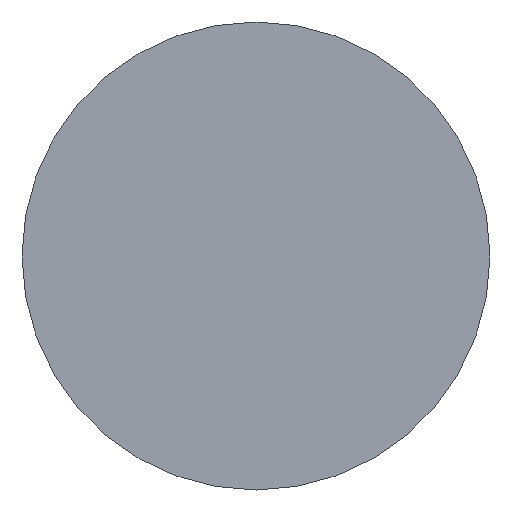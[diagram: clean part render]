
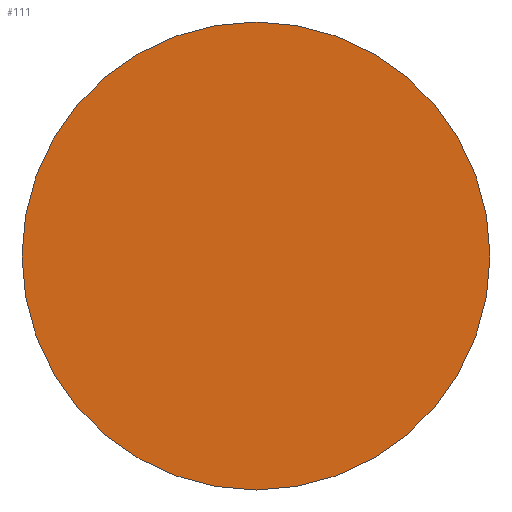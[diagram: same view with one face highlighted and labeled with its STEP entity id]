
A CAD part, left-side view. The second image highlights one B-rep face of the part: STEP entity #111.
In plain terms, the highlighted planar face has unit normal (-1, 0, 0).
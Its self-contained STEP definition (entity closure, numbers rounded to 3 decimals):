
#5 = DIRECTION ( 'NONE',  ( 1., 0., 0. ) ) ;
#15 = DIRECTION ( 'NONE',  ( 1., 0., 0. ) ) ;
#19 = CARTESIAN_POINT ( 'NONE',  ( -418.672, 34.658, 21.5 ) ) ;
#20 = CIRCLE ( 'NONE', #144, 3. ) ;
#22 = DIRECTION ( 'NONE',  ( 0., 0., 1. ) ) ;
#29 = VERTEX_POINT ( 'NONE', #68 ) ;
#35 = DIRECTION ( 'NONE',  ( -1., 0., 0. ) ) ;
#36 = AXIS2_PLACEMENT_3D ( 'NONE', #19, #5, #22 ) ;
#44 = EDGE_LOOP ( 'NONE', ( #69, #57 ) ) ;
#57 = ORIENTED_EDGE ( 'NONE', *, *, #66, .F. ) ;
#60 = PLANE ( 'NONE',  #78 ) ;
#66 = EDGE_CURVE ( 'NONE', #29, #102, #20, .T. ) ;
#68 = CARTESIAN_POINT ( 'NONE',  ( -418.672, 34.658, 18.5 ) ) ;
#69 = ORIENTED_EDGE ( 'NONE', *, *, #104, .F. ) ;
#78 = AXIS2_PLACEMENT_3D ( 'NONE', #125, #35, #117 ) ;
#88 = DIRECTION ( 'NONE',  ( 0., 0., 1. ) ) ;
#101 = CIRCLE ( 'NONE', #36, 3. ) ;
#102 = VERTEX_POINT ( 'NONE', #155 ) ;
#104 = EDGE_CURVE ( 'NONE', #102, #29, #101, .T. ) ;
#111 = ADVANCED_FACE ( 'NONE', ( #151 ), #60, .T. ) ;
#117 = DIRECTION ( 'NONE',  ( 0., 0., 1. ) ) ;
#125 = CARTESIAN_POINT ( 'NONE',  ( -418.672, 34.658, 21.5 ) ) ;
#144 = AXIS2_PLACEMENT_3D ( 'NONE', #145, #15, #88 ) ;
#145 = CARTESIAN_POINT ( 'NONE',  ( -418.672, 34.658, 21.5 ) ) ;
#151 = FACE_OUTER_BOUND ( 'NONE', #44, .T. ) ;
#155 = CARTESIAN_POINT ( 'NONE',  ( -418.672, 34.658, 24.5 ) ) ;
